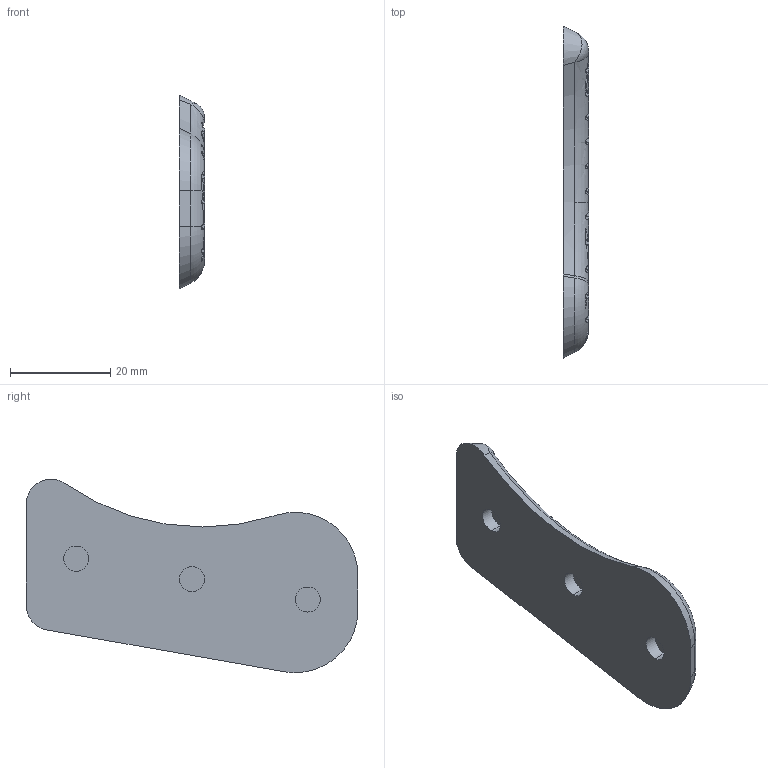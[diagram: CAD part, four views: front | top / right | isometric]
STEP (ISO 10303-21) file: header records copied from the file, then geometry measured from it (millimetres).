
FILE_DESCRIPTION (( 'STEP AP214' ), '1' );
FILE_NAME ('Grip_Thickener_Left.STEP', '2014-02-20T01:47:26', ( '' ), ( '' ), 'SwSTEP 2.0', 'SolidWorks 2013', '' );
FILE_SCHEMA (( 'AUTOMOTIVE_DESIGN' ));
Length unit declared in the file: millimetre
Products named in the file (1): Grip_Thickener_Left
Bounding box: 5.01 x 66.21 x 38.6 mm (x, y, z)
Volume: 7305.6 mm3; surface area: 4413.1 mm2
Topology: 1 solids, 1 shells, 220 faces, 582 edges, 368 vertices
Faces by surface type: cylinder 145, plane 57, torus 10, cone 6, bspline 2
Entity records: 8964 total; most frequent: CARTESIAN_POINT 4288, ORIENTED_EDGE 1164, DIRECTION 766, EDGE_CURVE 582, VERTEX_POINT 368, AXIS2_PLACEMENT_3D 270, LINE 226, VECTOR 226
